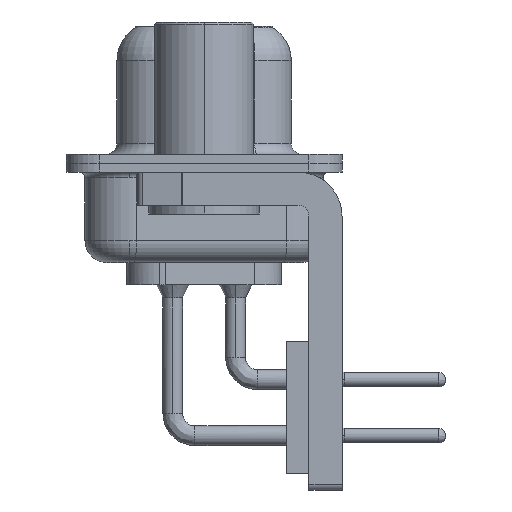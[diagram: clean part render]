
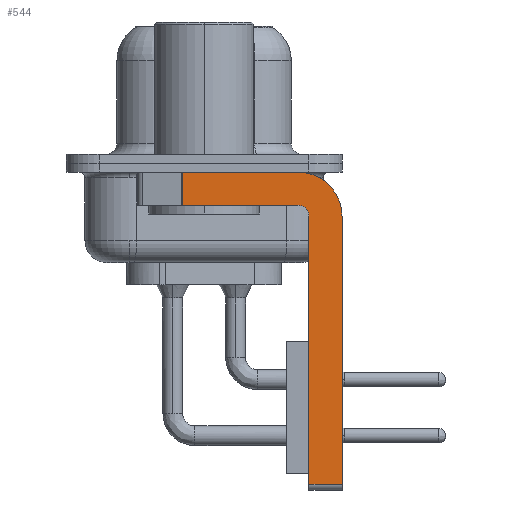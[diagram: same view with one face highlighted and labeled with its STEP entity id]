
A CAD part, left-side view. The second image highlights one B-rep face of the part: STEP entity #544.
In plain terms, the highlighted planar face has unit normal (-1, 0, 0).
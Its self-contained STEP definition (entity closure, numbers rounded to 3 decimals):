
#85 = DIRECTION ( 'NONE',  ( -1., 0., 0. ) ) ;
#483 = CARTESIAN_POINT ( 'NONE',  ( -2.9, -6.25, -14.55 ) ) ;
#544 = ADVANCED_FACE ( 'NONE', ( #20024 ), #6021, .F. ) ;
#672 = CARTESIAN_POINT ( 'NONE',  ( -2.9, -4.75, -2.4 ) ) ;
#1201 = DIRECTION ( 'NONE',  ( 0., -1., 0. ) ) ;
#1703 = VERTEX_POINT ( 'NONE', #30967 ) ;
#1934 = VECTOR ( 'NONE', #18580, 1000. ) ;
#2235 = VERTEX_POINT ( 'NONE', #483 ) ;
#2303 = CIRCLE ( 'NONE', #28860, 0.5 ) ;
#2545 = LINE ( 'NONE', #2702, #21366 ) ;
#2702 = CARTESIAN_POINT ( 'NONE',  ( -2.9, -4.25, -1.9 ) ) ;
#2812 = LINE ( 'NONE', #22506, #22389 ) ;
#2884 = CARTESIAN_POINT ( 'NONE',  ( -2.9, -6.25, -2.4 ) ) ;
#4016 = EDGE_CURVE ( 'NONE', #14057, #31500, #14593, .T. ) ;
#5046 = DIRECTION ( 'NONE',  ( 0., 1., 0. ) ) ;
#5796 = CARTESIAN_POINT ( 'NONE',  ( -2.9, -4.25, -2.4 ) ) ;
#6021 = PLANE ( 'NONE',  #30740 ) ;
#6135 = DIRECTION ( 'NONE',  ( 1., 0., 0. ) ) ;
#6396 = EDGE_CURVE ( 'NONE', #21969, #1703, #2545, .T. ) ;
#6724 = ORIENTED_EDGE ( 'NONE', *, *, #17655, .F. ) ;
#6828 = CARTESIAN_POINT ( 'NONE',  ( -2.9, -4.25, -2.4 ) ) ;
#6842 = VERTEX_POINT ( 'NONE', #24579 ) ;
#7809 = DIRECTION ( 'NONE',  ( 0., 0., -1. ) ) ;
#7915 = ORIENTED_EDGE ( 'NONE', *, *, #17712, .F. ) ;
#8597 = CARTESIAN_POINT ( 'NONE',  ( -2.9, 0.978, -0.4 ) ) ;
#8834 = VECTOR ( 'NONE', #12829, 1000. ) ;
#8947 = VERTEX_POINT ( 'NONE', #672 ) ;
#9203 = ORIENTED_EDGE ( 'NONE', *, *, #4016, .F. ) ;
#9225 = LINE ( 'NONE', #21011, #1934 ) ;
#9301 = DIRECTION ( 'NONE',  ( 0., 0., -1. ) ) ;
#9733 = EDGE_CURVE ( 'NONE', #31090, #2235, #9225, .T. ) ;
#11602 = CARTESIAN_POINT ( 'NONE',  ( -2.9, -4.75, -14.8 ) ) ;
#12829 = DIRECTION ( 'NONE',  ( 0., -1., 0. ) ) ;
#14052 = DIRECTION ( 'NONE',  ( 0., 0., 1. ) ) ;
#14057 = VERTEX_POINT ( 'NONE', #8597 ) ;
#14593 = LINE ( 'NONE', #27455, #8834 ) ;
#14811 = CARTESIAN_POINT ( 'NONE',  ( -2.9, -4.25, -2.4 ) ) ;
#14970 = ORIENTED_EDGE ( 'NONE', *, *, #15585, .T. ) ;
#15040 = VECTOR ( 'NONE', #1201, 1000. ) ;
#15585 = EDGE_CURVE ( 'NONE', #6842, #2235, #21562, .T. ) ;
#16127 = CARTESIAN_POINT ( 'NONE',  ( -2.9, -4.25, -14.55 ) ) ;
#16549 = DIRECTION ( 'NONE',  ( 0., 0., -1. ) ) ;
#17275 = DIRECTION ( 'NONE',  ( 0., 0., 1. ) ) ;
#17655 = EDGE_CURVE ( 'NONE', #6842, #8947, #23138, .T. ) ;
#17712 = EDGE_CURVE ( 'NONE', #31500, #31090, #26577, .T. ) ;
#18533 = CARTESIAN_POINT ( 'NONE',  ( -2.9, -4.25, -1.9 ) ) ;
#18580 = DIRECTION ( 'NONE',  ( 0., 0., -1. ) ) ;
#19596 = EDGE_CURVE ( 'NONE', #8947, #21969, #2303, .T. ) ;
#19772 = ORIENTED_EDGE ( 'NONE', *, *, #6396, .F. ) ;
#20024 = FACE_OUTER_BOUND ( 'NONE', #21826, .T. ) ;
#20578 = AXIS2_PLACEMENT_3D ( 'NONE', #6828, #23982, #9301 ) ;
#21011 = CARTESIAN_POINT ( 'NONE',  ( -2.9, -6.25, -2.4 ) ) ;
#21366 = VECTOR ( 'NONE', #5046, 1000. ) ;
#21562 = LINE ( 'NONE', #16127, #15040 ) ;
#21826 = EDGE_LOOP ( 'NONE', ( #9203, #25292, #19772, #28364, #6724, #14970, #28518, #7915 ) ) ;
#21969 = VERTEX_POINT ( 'NONE', #18533 ) ;
#22389 = VECTOR ( 'NONE', #7809, 1000. ) ;
#22506 = CARTESIAN_POINT ( 'NONE',  ( -2.9, 0.978, -1.9 ) ) ;
#23138 = LINE ( 'NONE', #11602, #27335 ) ;
#23982 = DIRECTION ( 'NONE',  ( 1., 0., 0. ) ) ;
#24579 = CARTESIAN_POINT ( 'NONE',  ( -2.9, -4.75, -14.55 ) ) ;
#25292 = ORIENTED_EDGE ( 'NONE', *, *, #26451, .T. ) ;
#26451 = EDGE_CURVE ( 'NONE', #14057, #1703, #2812, .T. ) ;
#26577 = CIRCLE ( 'NONE', #20578, 2. ) ;
#26916 = CARTESIAN_POINT ( 'NONE',  ( -2.9, -4.25, -0.4 ) ) ;
#27335 = VECTOR ( 'NONE', #14052, 1000. ) ;
#27455 = CARTESIAN_POINT ( 'NONE',  ( -2.9, 3., -0.4 ) ) ;
#28364 = ORIENTED_EDGE ( 'NONE', *, *, #19596, .F. ) ;
#28518 = ORIENTED_EDGE ( 'NONE', *, *, #9733, .F. ) ;
#28860 = AXIS2_PLACEMENT_3D ( 'NONE', #14811, #85, #17275 ) ;
#30740 = AXIS2_PLACEMENT_3D ( 'NONE', #5796, #6135, #16549 ) ;
#30967 = CARTESIAN_POINT ( 'NONE',  ( -2.9, 0.978, -1.9 ) ) ;
#31090 = VERTEX_POINT ( 'NONE', #2884 ) ;
#31500 = VERTEX_POINT ( 'NONE', #26916 ) ;
